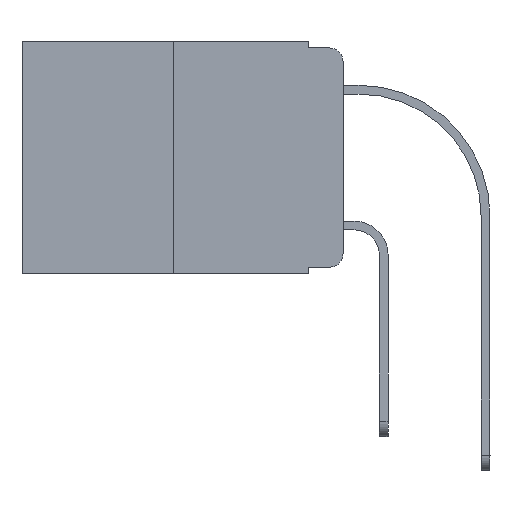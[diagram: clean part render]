
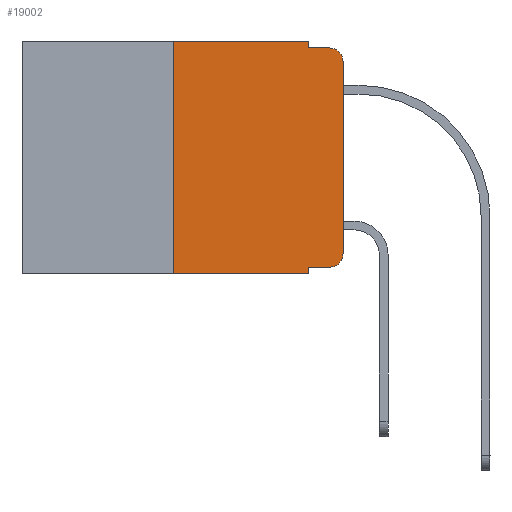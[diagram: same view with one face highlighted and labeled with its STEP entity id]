
A CAD part, left-side view. The second image highlights one B-rep face of the part: STEP entity #19002.
In plain terms, the highlighted planar face has unit normal (-1, 0, 0).
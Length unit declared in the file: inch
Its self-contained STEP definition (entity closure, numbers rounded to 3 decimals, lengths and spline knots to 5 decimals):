
#316 = VERTEX_POINT ( 'NONE', #20101 ) ;
#666 = EDGE_CURVE ( 'NONE', #21982, #14716, #3316, .T. ) ;
#904 = VECTOR ( 'NONE', #6916, 39.37008 ) ;
#1859 = AXIS2_PLACEMENT_3D ( 'NONE', #11687, #18831, #2769 ) ;
#2348 = LINE ( 'NONE', #20160, #21893 ) ;
#2586 = DIRECTION ( 'NONE',  ( 0., -1., 0. ) ) ;
#2769 = DIRECTION ( 'NONE',  ( 0., 0., -1. ) ) ;
#2890 = DIRECTION ( 'NONE',  ( 0., 0., -1. ) ) ;
#3022 = ORIENTED_EDGE ( 'NONE', *, *, #11261, .T. ) ;
#3161 = CARTESIAN_POINT ( 'NONE',  ( 0., 0., 0. ) ) ;
#3185 = VECTOR ( 'NONE', #2890, 39.37008 ) ;
#3316 = LINE ( 'NONE', #19623, #5240 ) ;
#3569 = FACE_OUTER_BOUND ( 'NONE', #11113, .T. ) ;
#3711 = CARTESIAN_POINT ( 'NONE',  ( 0., 0.051, 0. ) ) ;
#3872 = DIRECTION ( 'NONE',  ( 0., -1., 0. ) ) ;
#3911 = DIRECTION ( 'NONE',  ( 0., 0., -1. ) ) ;
#4003 = CARTESIAN_POINT ( 'NONE',  ( 0., 0., -0.313 ) ) ;
#4556 = LINE ( 'NONE', #20861, #904 ) ;
#4619 = ORIENTED_EDGE ( 'NONE', *, *, #16767, .T. ) ;
#4758 = LINE ( 'NONE', #19064, #3185 ) ;
#5240 = VECTOR ( 'NONE', #10479, 39.37008 ) ;
#5669 = CARTESIAN_POINT ( 'NONE',  ( 0., 0.02, -0.313 ) ) ;
#5814 = EDGE_CURVE ( 'NONE', #17546, #14716, #13385, .T. ) ;
#6577 = VECTOR ( 'NONE', #22764, 39.37008 ) ;
#6686 = LINE ( 'NONE', #8458, #13788 ) ;
#6736 = DIRECTION ( 'NONE',  ( 1., 0., 0. ) ) ;
#6916 = DIRECTION ( 'NONE',  ( 0., -1., 0. ) ) ;
#7483 = EDGE_CURVE ( 'NONE', #316, #15885, #4556, .T. ) ;
#7689 = CARTESIAN_POINT ( 'NONE',  ( 0., 0.25, 0. ) ) ;
#8003 = EDGE_CURVE ( 'NONE', #16812, #316, #4758, .T. ) ;
#8458 = CARTESIAN_POINT ( 'NONE',  ( 0., 0.25, 0. ) ) ;
#9858 = VECTOR ( 'NONE', #2586, 39.37008 ) ;
#9885 = CARTESIAN_POINT ( 'NONE',  ( 0., 0.473, -0.343 ) ) ;
#10252 = CIRCLE ( 'NONE', #12887, 0.02 ) ;
#10479 = DIRECTION ( 'NONE',  ( 0., 0., -1. ) ) ;
#11113 = EDGE_LOOP ( 'NONE', ( #4619, #18686, #11326, #14847, #16789, #14230, #22701, #11733, #18522, #3022 ) ) ;
#11143 = CARTESIAN_POINT ( 'NONE',  ( 0., 0.051, -0.343 ) ) ;
#11261 = EDGE_CURVE ( 'NONE', #20360, #17889, #10252, .T. ) ;
#11326 = ORIENTED_EDGE ( 'NONE', *, *, #7483, .F. ) ;
#11687 = CARTESIAN_POINT ( 'NONE',  ( 0., 0.02, -0.03 ) ) ;
#11733 = ORIENTED_EDGE ( 'NONE', *, *, #666, .F. ) ;
#11972 = CIRCLE ( 'NONE', #1859, 0.02 ) ;
#12036 = VERTEX_POINT ( 'NONE', #22509 ) ;
#12824 = DIRECTION ( 'NONE',  ( -1., 0., 0. ) ) ;
#12887 = AXIS2_PLACEMENT_3D ( 'NONE', #5669, #12824, #3911 ) ;
#13234 = EDGE_CURVE ( 'NONE', #21982, #20360, #22878, .T. ) ;
#13381 = EDGE_CURVE ( 'NONE', #13855, #16812, #2348, .T. ) ;
#13385 = LINE ( 'NONE', #9885, #9858 ) ;
#13788 = VECTOR ( 'NONE', #13835, 39.37008 ) ;
#13835 = DIRECTION ( 'NONE',  ( 0., 0., 1. ) ) ;
#13855 = VERTEX_POINT ( 'NONE', #7689 ) ;
#14230 = ORIENTED_EDGE ( 'NONE', *, *, #20691, .F. ) ;
#14716 = VERTEX_POINT ( 'NONE', #11143 ) ;
#14847 = ORIENTED_EDGE ( 'NONE', *, *, #8003, .F. ) ;
#15809 = CARTESIAN_POINT ( 'NONE',  ( 0., 0.02, -0.333 ) ) ;
#15885 = VERTEX_POINT ( 'NONE', #17952 ) ;
#16455 = VECTOR ( 'NONE', #22834, 39.37008 ) ;
#16767 = EDGE_CURVE ( 'NONE', #17889, #12036, #17354, .T. ) ;
#16789 = ORIENTED_EDGE ( 'NONE', *, *, #13381, .F. ) ;
#16812 = VERTEX_POINT ( 'NONE', #3711 ) ;
#16878 = AXIS2_PLACEMENT_3D ( 'NONE', #23031, #6736, #17869 ) ;
#16933 = CARTESIAN_POINT ( 'NONE',  ( 0., 0.051, -0.333 ) ) ;
#17354 = LINE ( 'NONE', #3161, #16455 ) ;
#17546 = VERTEX_POINT ( 'NONE', #18580 ) ;
#17869 = DIRECTION ( 'NONE',  ( 0., 0., -1. ) ) ;
#17889 = VERTEX_POINT ( 'NONE', #4003 ) ;
#17952 = CARTESIAN_POINT ( 'NONE',  ( 0., 0.02, -0.01 ) ) ;
#18522 = ORIENTED_EDGE ( 'NONE', *, *, #13234, .T. ) ;
#18580 = CARTESIAN_POINT ( 'NONE',  ( 0., 0.25, -0.343 ) ) ;
#18686 = ORIENTED_EDGE ( 'NONE', *, *, #21631, .T. ) ;
#18831 = DIRECTION ( 'NONE',  ( -1., 0., 0. ) ) ;
#19002 = ADVANCED_FACE ( 'NONE', ( #3569 ), #22912, .F. ) ;
#19064 = CARTESIAN_POINT ( 'NONE',  ( 0., 0.051, 0. ) ) ;
#19623 = CARTESIAN_POINT ( 'NONE',  ( 0., 0.051, 0. ) ) ;
#20101 = CARTESIAN_POINT ( 'NONE',  ( 0., 0.051, -0.01 ) ) ;
#20160 = CARTESIAN_POINT ( 'NONE',  ( 0., 0.473, 0. ) ) ;
#20360 = VERTEX_POINT ( 'NONE', #15809 ) ;
#20691 = EDGE_CURVE ( 'NONE', #17546, #13855, #6686, .T. ) ;
#20861 = CARTESIAN_POINT ( 'NONE',  ( 0., 0.051, -0.01 ) ) ;
#21012 = CARTESIAN_POINT ( 'NONE',  ( 0., 0.051, -0.333 ) ) ;
#21631 = EDGE_CURVE ( 'NONE', #12036, #15885, #11972, .T. ) ;
#21893 = VECTOR ( 'NONE', #3872, 39.37008 ) ;
#21982 = VERTEX_POINT ( 'NONE', #16933 ) ;
#22509 = CARTESIAN_POINT ( 'NONE',  ( 0., 0., -0.03 ) ) ;
#22701 = ORIENTED_EDGE ( 'NONE', *, *, #5814, .T. ) ;
#22764 = DIRECTION ( 'NONE',  ( 0., -1., 0. ) ) ;
#22834 = DIRECTION ( 'NONE',  ( 0., 0., 1. ) ) ;
#22878 = LINE ( 'NONE', #21012, #6577 ) ;
#22912 = PLANE ( 'NONE',  #16878 ) ;
#23031 = CARTESIAN_POINT ( 'NONE',  ( 0., 0.473, 0. ) ) ;
